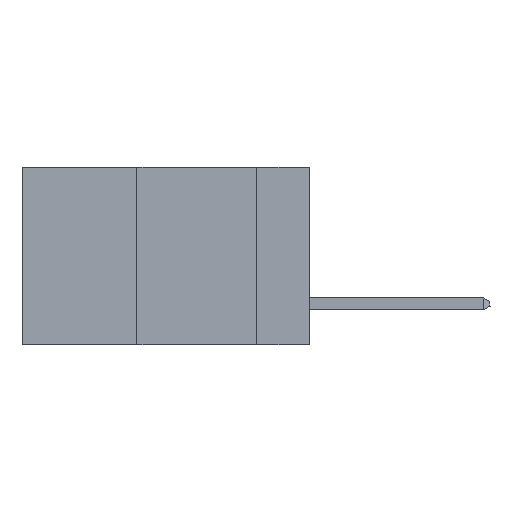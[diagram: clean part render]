
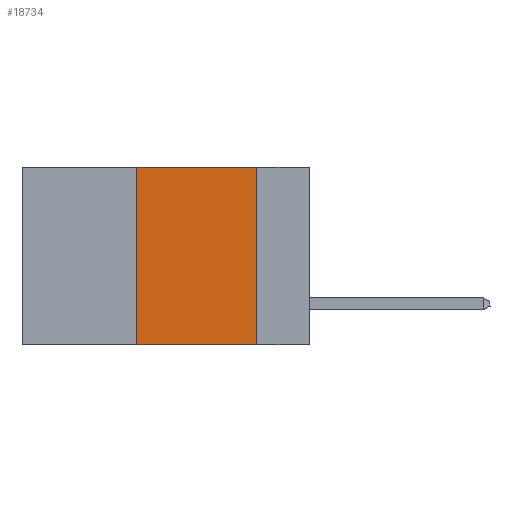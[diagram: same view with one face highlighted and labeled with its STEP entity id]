
A CAD part, left-side view. The second image highlights one B-rep face of the part: STEP entity #18734.
In plain terms, the highlighted planar face has unit normal (-1, 0, 0).
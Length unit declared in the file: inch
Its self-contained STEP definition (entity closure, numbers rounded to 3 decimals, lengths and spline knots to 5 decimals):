
#68 = LINE ( 'NONE', #11129, #13035 ) ;
#422 = DIRECTION ( 'NONE',  ( 1., 0., 0. ) ) ;
#933 = VERTEX_POINT ( 'NONE', #15381 ) ;
#1139 = CARTESIAN_POINT ( 'NONE',  ( 0., 0.11, -0.37 ) ) ;
#1210 = ORIENTED_EDGE ( 'NONE', *, *, #18797, .F. ) ;
#1279 = CARTESIAN_POINT ( 'NONE',  ( 0., 0.36, 0. ) ) ;
#2506 = DIRECTION ( 'NONE',  ( 0., -1., 0. ) ) ;
#3400 = DIRECTION ( 'NONE',  ( 0., 0., 1. ) ) ;
#3703 = CARTESIAN_POINT ( 'NONE',  ( 0., 0.36, 0. ) ) ;
#3951 = CARTESIAN_POINT ( 'NONE',  ( 0., 0.6, -0.37 ) ) ;
#5357 = EDGE_CURVE ( 'NONE', #933, #10446, #68, .T. ) ;
#5656 = CARTESIAN_POINT ( 'NONE',  ( 0., 0.6, 0. ) ) ;
#5831 = EDGE_CURVE ( 'NONE', #8682, #10446, #8337, .T. ) ;
#5981 = ORIENTED_EDGE ( 'NONE', *, *, #5831, .T. ) ;
#7537 = VECTOR ( 'NONE', #3400, 39.37008 ) ;
#8317 = LINE ( 'NONE', #21079, #19552 ) ;
#8337 = LINE ( 'NONE', #3951, #18266 ) ;
#8682 = VERTEX_POINT ( 'NONE', #16915 ) ;
#10446 = VERTEX_POINT ( 'NONE', #1139 ) ;
#11024 = ORIENTED_EDGE ( 'NONE', *, *, #5357, .F. ) ;
#11129 = CARTESIAN_POINT ( 'NONE',  ( 0., 0.11, 0. ) ) ;
#11567 = ORIENTED_EDGE ( 'NONE', *, *, #17530, .F. ) ;
#11743 = LINE ( 'NONE', #3703, #7537 ) ;
#12240 = FACE_OUTER_BOUND ( 'NONE', #16433, .T. ) ;
#12423 = DIRECTION ( 'NONE',  ( 0., 0., -1. ) ) ;
#13035 = VECTOR ( 'NONE', #16430, 39.37008 ) ;
#13359 = AXIS2_PLACEMENT_3D ( 'NONE', #5656, #422, #12423 ) ;
#15381 = CARTESIAN_POINT ( 'NONE',  ( 0., 0.11, 0. ) ) ;
#15793 = PLANE ( 'NONE',  #13359 ) ;
#16430 = DIRECTION ( 'NONE',  ( 0., 0., -1. ) ) ;
#16433 = EDGE_LOOP ( 'NONE', ( #11024, #1210, #11567, #5981 ) ) ;
#16915 = CARTESIAN_POINT ( 'NONE',  ( 0., 0.36, -0.37 ) ) ;
#17530 = EDGE_CURVE ( 'NONE', #8682, #18444, #11743, .T. ) ;
#18266 = VECTOR ( 'NONE', #19158, 39.37008 ) ;
#18444 = VERTEX_POINT ( 'NONE', #1279 ) ;
#18734 = ADVANCED_FACE ( 'NONE', ( #12240 ), #15793, .F. ) ;
#18797 = EDGE_CURVE ( 'NONE', #18444, #933, #8317, .T. ) ;
#19158 = DIRECTION ( 'NONE',  ( 0., -1., 0. ) ) ;
#19552 = VECTOR ( 'NONE', #2506, 39.37008 ) ;
#21079 = CARTESIAN_POINT ( 'NONE',  ( 0., 0.6, 0. ) ) ;
